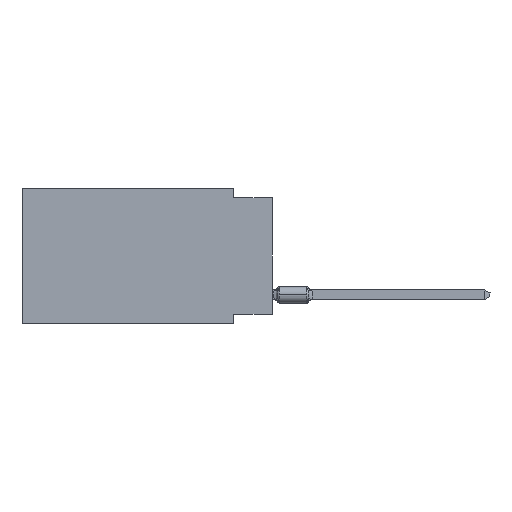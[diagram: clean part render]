
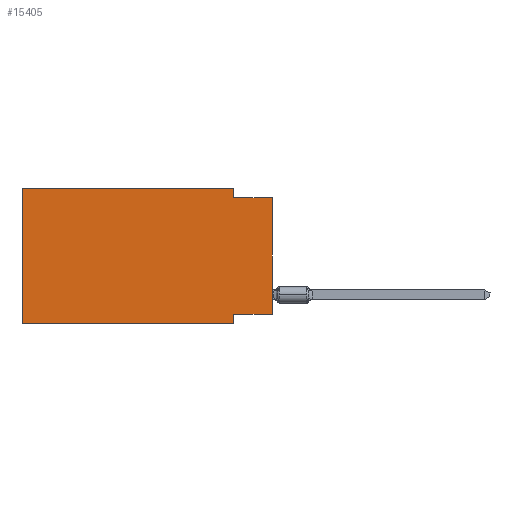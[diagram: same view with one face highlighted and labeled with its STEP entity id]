
A CAD part, left-side view. The second image highlights one B-rep face of the part: STEP entity #15405.
In plain terms, the highlighted planar face has unit normal (-1, 0, 0).
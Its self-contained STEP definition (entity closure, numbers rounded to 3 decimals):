
#667 = LINE ( 'NONE', #42441, #25099 ) ;
#835 = EDGE_CURVE ( 'NONE', #11877, #15975, #26496, .T. ) ;
#2662 = DIRECTION ( 'NONE',  ( 0., -1., 0. ) ) ;
#3936 = CARTESIAN_POINT ( 'NONE',  ( 0., 16.383, -8.89 ) ) ;
#5250 = VECTOR ( 'NONE', #38654, 1000. ) ;
#5365 = ORIENTED_EDGE ( 'NONE', *, *, #21685, .F. ) ;
#5500 = CARTESIAN_POINT ( 'NONE',  ( 0., 0., -8.255 ) ) ;
#6881 = ORIENTED_EDGE ( 'NONE', *, *, #45048, .F. ) ;
#6976 = DIRECTION ( 'NONE',  ( 0., -1., 0. ) ) ;
#7245 = EDGE_CURVE ( 'NONE', #15975, #24670, #41467, .T. ) ;
#8736 = VECTOR ( 'NONE', #2662, 1000. ) ;
#9854 = EDGE_CURVE ( 'NONE', #17921, #13256, #20662, .T. ) ;
#10412 = CARTESIAN_POINT ( 'NONE',  ( 0., 0., -0.635 ) ) ;
#11161 = DIRECTION ( 'NONE',  ( 0., 0., 1. ) ) ;
#11877 = VERTEX_POINT ( 'NONE', #13153 ) ;
#12885 = AXIS2_PLACEMENT_3D ( 'NONE', #19884, #27876, #34490 ) ;
#13153 = CARTESIAN_POINT ( 'NONE',  ( 0., 16.383, -8.89 ) ) ;
#13256 = VERTEX_POINT ( 'NONE', #44428 ) ;
#13809 = ORIENTED_EDGE ( 'NONE', *, *, #25301, .F. ) ;
#14164 = CARTESIAN_POINT ( 'NONE',  ( 0., 2.54, -0.635 ) ) ;
#14594 = CARTESIAN_POINT ( 'NONE',  ( 0., 0., -0.635 ) ) ;
#15405 = ADVANCED_FACE ( 'NONE', ( #41780 ), #41320, .F. ) ;
#15831 = VERTEX_POINT ( 'NONE', #14164 ) ;
#15975 = VERTEX_POINT ( 'NONE', #21711 ) ;
#17696 = EDGE_CURVE ( 'NONE', #17921, #27084, #667, .T. ) ;
#17867 = DIRECTION ( 'NONE',  ( 0., -1., 0. ) ) ;
#17921 = VERTEX_POINT ( 'NONE', #5500 ) ;
#18097 = CARTESIAN_POINT ( 'NONE',  ( 0., 2.54, 0. ) ) ;
#18619 = VERTEX_POINT ( 'NONE', #35572 ) ;
#18998 = ORIENTED_EDGE ( 'NONE', *, *, #32218, .T. ) ;
#19884 = CARTESIAN_POINT ( 'NONE',  ( 0., 16.383, 0. ) ) ;
#20662 = LINE ( 'NONE', #20864, #5250 ) ;
#20858 = DIRECTION ( 'NONE',  ( 0., 0., -1. ) ) ;
#20864 = CARTESIAN_POINT ( 'NONE',  ( 0., 0., -8.255 ) ) ;
#21685 = EDGE_CURVE ( 'NONE', #24670, #15831, #28839, .T. ) ;
#21711 = CARTESIAN_POINT ( 'NONE',  ( 0., 16.383, 0. ) ) ;
#22350 = EDGE_LOOP ( 'NONE', ( #35275, #13809, #5365, #43016, #33454, #18998, #6881, #22693 ) ) ;
#22693 = ORIENTED_EDGE ( 'NONE', *, *, #9854, .F. ) ;
#24670 = VERTEX_POINT ( 'NONE', #38312 ) ;
#25099 = VECTOR ( 'NONE', #11161, 1000. ) ;
#25301 = EDGE_CURVE ( 'NONE', #15831, #27084, #41070, .T. ) ;
#25935 = VECTOR ( 'NONE', #17867, 1000. ) ;
#26496 = LINE ( 'NONE', #43571, #38008 ) ;
#27084 = VERTEX_POINT ( 'NONE', #14594 ) ;
#27876 = DIRECTION ( 'NONE',  ( 1., 0., 0. ) ) ;
#27946 = LINE ( 'NONE', #35441, #37128 ) ;
#28839 = LINE ( 'NONE', #18097, #40835 ) ;
#29449 = DIRECTION ( 'NONE',  ( 0., 0., 1. ) ) ;
#32218 = EDGE_CURVE ( 'NONE', #11877, #18619, #38633, .T. ) ;
#33454 = ORIENTED_EDGE ( 'NONE', *, *, #835, .F. ) ;
#34232 = VECTOR ( 'NONE', #6976, 1000. ) ;
#34490 = DIRECTION ( 'NONE',  ( 0., 0., -1. ) ) ;
#35234 = DIRECTION ( 'NONE',  ( 0., 0., -1. ) ) ;
#35275 = ORIENTED_EDGE ( 'NONE', *, *, #17696, .T. ) ;
#35441 = CARTESIAN_POINT ( 'NONE',  ( 0., 2.54, -8.89 ) ) ;
#35572 = CARTESIAN_POINT ( 'NONE',  ( 0., 2.54, -8.89 ) ) ;
#37128 = VECTOR ( 'NONE', #20858, 1000. ) ;
#37375 = CARTESIAN_POINT ( 'NONE',  ( 0., 16.383, 0. ) ) ;
#38008 = VECTOR ( 'NONE', #29449, 1000. ) ;
#38312 = CARTESIAN_POINT ( 'NONE',  ( 0., 2.54, 0. ) ) ;
#38633 = LINE ( 'NONE', #3936, #25935 ) ;
#38654 = DIRECTION ( 'NONE',  ( 0., 1., 0. ) ) ;
#40835 = VECTOR ( 'NONE', #35234, 1000. ) ;
#41070 = LINE ( 'NONE', #10412, #34232 ) ;
#41320 = PLANE ( 'NONE',  #12885 ) ;
#41467 = LINE ( 'NONE', #37375, #8736 ) ;
#41780 = FACE_OUTER_BOUND ( 'NONE', #22350, .T. ) ;
#42441 = CARTESIAN_POINT ( 'NONE',  ( 0., 0., 0. ) ) ;
#43016 = ORIENTED_EDGE ( 'NONE', *, *, #7245, .F. ) ;
#43571 = CARTESIAN_POINT ( 'NONE',  ( 0., 16.383, 0. ) ) ;
#44428 = CARTESIAN_POINT ( 'NONE',  ( 0., 2.54, -8.255 ) ) ;
#45048 = EDGE_CURVE ( 'NONE', #13256, #18619, #27946, .T. ) ;
